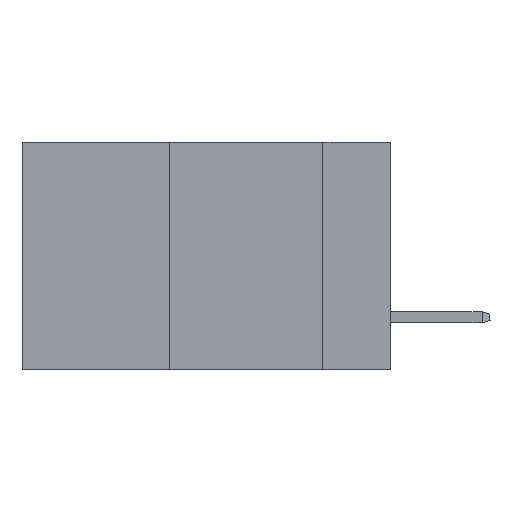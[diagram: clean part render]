
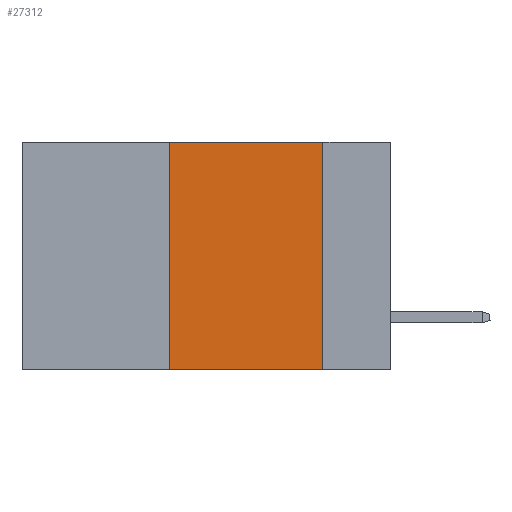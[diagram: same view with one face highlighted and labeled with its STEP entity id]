
A CAD part, left-side view. The second image highlights one B-rep face of the part: STEP entity #27312.
In plain terms, the highlighted planar face has unit normal (-1, 0, 0).
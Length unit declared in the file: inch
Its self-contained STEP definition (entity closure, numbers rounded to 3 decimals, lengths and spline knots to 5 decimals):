
#14 = VERTEX_POINT ( 'NONE', #30791 ) ;
#183 = EDGE_CURVE ( 'NONE', #14, #15151, #5940, .T. ) ;
#579 = VERTEX_POINT ( 'NONE', #1441 ) ;
#1031 = DIRECTION ( 'NONE',  ( 0., -1., 0. ) ) ;
#1131 = CARTESIAN_POINT ( 'NONE',  ( 0., 0.6, 0. ) ) ;
#1441 = CARTESIAN_POINT ( 'NONE',  ( 0., 0.11, -0.37 ) ) ;
#1927 = VECTOR ( 'NONE', #33956, 39.37008 ) ;
#3104 = EDGE_CURVE ( 'NONE', #34204, #14, #14480, .T. ) ;
#3193 = ORIENTED_EDGE ( 'NONE', *, *, #3104, .F. ) ;
#3796 = DIRECTION ( 'NONE',  ( 0., -1., 0. ) ) ;
#5106 = VECTOR ( 'NONE', #3796, 39.37008 ) ;
#5940 = LINE ( 'NONE', #1131, #5106 ) ;
#7173 = PLANE ( 'NONE',  #12740 ) ;
#7413 = ORIENTED_EDGE ( 'NONE', *, *, #183, .F. ) ;
#9184 = LINE ( 'NONE', #31410, #1927 ) ;
#9866 = CARTESIAN_POINT ( 'NONE',  ( 0., 0.11, 0. ) ) ;
#9913 = DIRECTION ( 'NONE',  ( 1., 0., 0. ) ) ;
#11129 = DIRECTION ( 'NONE',  ( 0., 0., 1. ) ) ;
#11189 = FACE_OUTER_BOUND ( 'NONE', #19562, .T. ) ;
#12740 = AXIS2_PLACEMENT_3D ( 'NONE', #15306, #9913, #28364 ) ;
#14480 = LINE ( 'NONE', #29218, #16239 ) ;
#15151 = VERTEX_POINT ( 'NONE', #9866 ) ;
#15306 = CARTESIAN_POINT ( 'NONE',  ( 0., 0.6, 0. ) ) ;
#16239 = VECTOR ( 'NONE', #11129, 39.37008 ) ;
#18432 = EDGE_CURVE ( 'NONE', #15151, #579, #9184, .T. ) ;
#18682 = LINE ( 'NONE', #32761, #21088 ) ;
#19562 = EDGE_LOOP ( 'NONE', ( #26043, #7413, #3193, #28393 ) ) ;
#21088 = VECTOR ( 'NONE', #1031, 39.37008 ) ;
#23830 = EDGE_CURVE ( 'NONE', #34204, #579, #18682, .T. ) ;
#26043 = ORIENTED_EDGE ( 'NONE', *, *, #18432, .F. ) ;
#27312 = ADVANCED_FACE ( 'NONE', ( #11189 ), #7173, .F. ) ;
#28364 = DIRECTION ( 'NONE',  ( 0., 0., -1. ) ) ;
#28393 = ORIENTED_EDGE ( 'NONE', *, *, #23830, .T. ) ;
#29218 = CARTESIAN_POINT ( 'NONE',  ( 0., 0.36, 0. ) ) ;
#30479 = CARTESIAN_POINT ( 'NONE',  ( 0., 0.36, -0.37 ) ) ;
#30791 = CARTESIAN_POINT ( 'NONE',  ( 0., 0.36, 0. ) ) ;
#31410 = CARTESIAN_POINT ( 'NONE',  ( 0., 0.11, 0. ) ) ;
#32761 = CARTESIAN_POINT ( 'NONE',  ( 0., 0.6, -0.37 ) ) ;
#33956 = DIRECTION ( 'NONE',  ( 0., 0., -1. ) ) ;
#34204 = VERTEX_POINT ( 'NONE', #30479 ) ;
